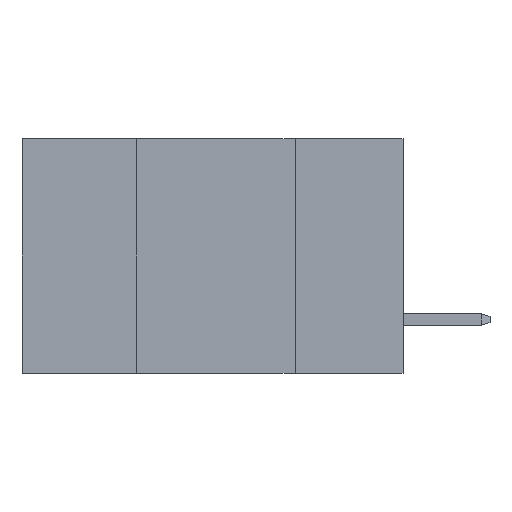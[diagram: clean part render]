
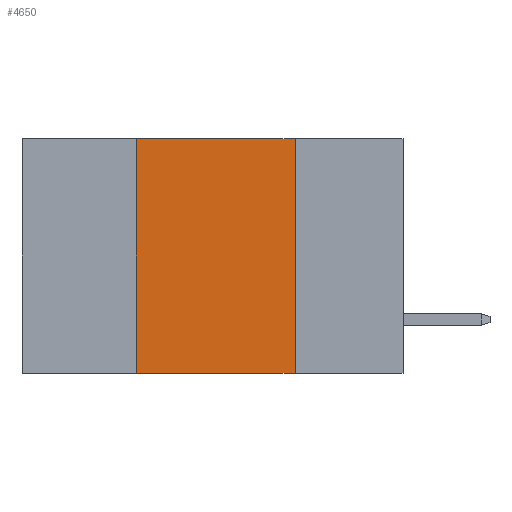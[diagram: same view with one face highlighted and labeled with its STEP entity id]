
A CAD part, left-side view. The second image highlights one B-rep face of the part: STEP entity #4650.
In plain terms, the highlighted planar face has unit normal (-1, 0, 0).
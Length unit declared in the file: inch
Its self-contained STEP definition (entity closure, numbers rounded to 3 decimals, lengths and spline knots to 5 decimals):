
#60 = EDGE_CURVE ( 'NONE', #7392, #739, #3875, .T. ) ;
#227 = ORIENTED_EDGE ( 'NONE', *, *, #4458, .F. ) ;
#739 = VERTEX_POINT ( 'NONE', #9825 ) ;
#1034 = DIRECTION ( 'NONE',  ( 0., 0., -1. ) ) ;
#1101 = CARTESIAN_POINT ( 'NONE',  ( 0., 0.6, 0. ) ) ;
#1130 = DIRECTION ( 'NONE',  ( 0., 0., -1. ) ) ;
#1355 = CARTESIAN_POINT ( 'NONE',  ( 0., 0.17, 0. ) ) ;
#1356 = VECTOR ( 'NONE', #6719, 39.37008 ) ;
#1893 = CARTESIAN_POINT ( 'NONE',  ( 0., 0.17, 0. ) ) ;
#1922 = DIRECTION ( 'NONE',  ( 1., 0., 0. ) ) ;
#3131 = CARTESIAN_POINT ( 'NONE',  ( 0., 0.42, 0. ) ) ;
#3298 = VERTEX_POINT ( 'NONE', #1355 ) ;
#3436 = VERTEX_POINT ( 'NONE', #9649 ) ;
#3466 = ORIENTED_EDGE ( 'NONE', *, *, #10875, .F. ) ;
#3875 = LINE ( 'NONE', #3131, #8969 ) ;
#4203 = VECTOR ( 'NONE', #7854, 39.37008 ) ;
#4458 = EDGE_CURVE ( 'NONE', #3298, #3436, #8987, .T. ) ;
#4540 = CARTESIAN_POINT ( 'NONE',  ( 0., 0.6, 0. ) ) ;
#4576 = PLANE ( 'NONE',  #6663 ) ;
#4650 = ADVANCED_FACE ( 'NONE', ( #5491 ), #4576, .F. ) ;
#5491 = FACE_OUTER_BOUND ( 'NONE', #5698, .T. ) ;
#5698 = EDGE_LOOP ( 'NONE', ( #227, #3466, #6156, #7184 ) ) ;
#5806 = LINE ( 'NONE', #9439, #1356 ) ;
#5956 = EDGE_CURVE ( 'NONE', #7392, #3436, #5806, .T. ) ;
#6156 = ORIENTED_EDGE ( 'NONE', *, *, #60, .F. ) ;
#6523 = DIRECTION ( 'NONE',  ( 0., 0., 1. ) ) ;
#6663 = AXIS2_PLACEMENT_3D ( 'NONE', #1101, #1922, #1034 ) ;
#6719 = DIRECTION ( 'NONE',  ( 0., -1., 0. ) ) ;
#7184 = ORIENTED_EDGE ( 'NONE', *, *, #5956, .T. ) ;
#7392 = VERTEX_POINT ( 'NONE', #11281 ) ;
#7854 = DIRECTION ( 'NONE',  ( 0., -1., 0. ) ) ;
#7916 = LINE ( 'NONE', #4540, #4203 ) ;
#8969 = VECTOR ( 'NONE', #6523, 39.37008 ) ;
#8987 = LINE ( 'NONE', #1893, #9747 ) ;
#9439 = CARTESIAN_POINT ( 'NONE',  ( 0., 0.6, -0.37 ) ) ;
#9649 = CARTESIAN_POINT ( 'NONE',  ( 0., 0.17, -0.37 ) ) ;
#9747 = VECTOR ( 'NONE', #1130, 39.37008 ) ;
#9825 = CARTESIAN_POINT ( 'NONE',  ( 0., 0.42, 0. ) ) ;
#10875 = EDGE_CURVE ( 'NONE', #739, #3298, #7916, .T. ) ;
#11281 = CARTESIAN_POINT ( 'NONE',  ( 0., 0.42, -0.37 ) ) ;
